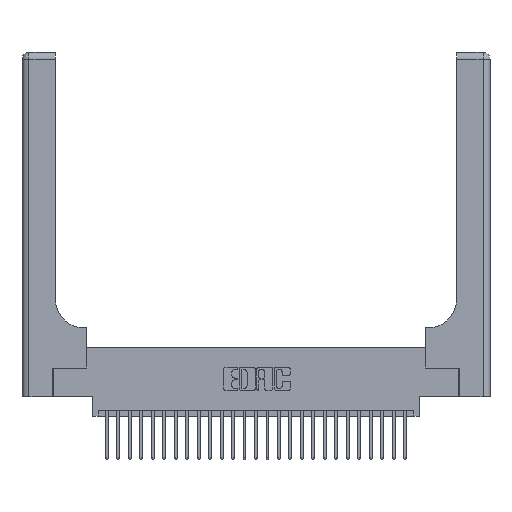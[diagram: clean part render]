
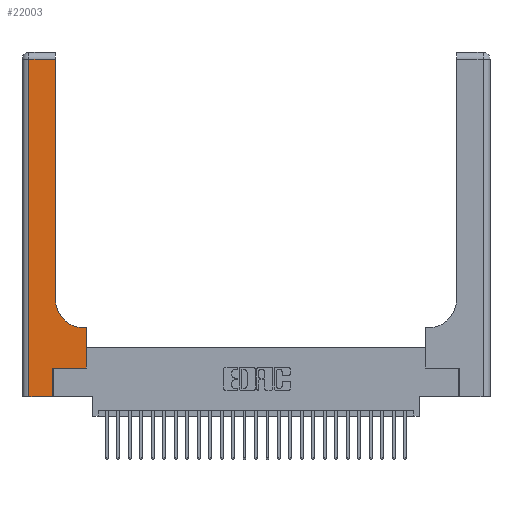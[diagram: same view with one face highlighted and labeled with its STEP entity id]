
A CAD part, top view. The second image highlights one B-rep face of the part: STEP entity #22003.
In plain terms, the highlighted planar face has unit normal (0, 0, 1).
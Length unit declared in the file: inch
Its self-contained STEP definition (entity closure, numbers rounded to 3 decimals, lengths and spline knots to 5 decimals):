
#26 = DIRECTION ( 'NONE',  ( 0., 0., -1. ) ) ;
#573 = CARTESIAN_POINT ( 'NONE',  ( 0.5415, 0.6, 0.37 ) ) ;
#865 = ORIENTED_EDGE ( 'NONE', *, *, #6812, .T. ) ;
#1028 = DIRECTION ( 'NONE',  ( -1., 0., 0. ) ) ;
#1281 = EDGE_CURVE ( 'NONE', #1864, #8788, #22745, .T. ) ;
#1453 = VERTEX_POINT ( 'NONE', #10189 ) ;
#1601 = VECTOR ( 'NONE', #24154, 39.37008 ) ;
#1743 = CARTESIAN_POINT ( 'NONE',  ( 0.2915, 3., 0.37 ) ) ;
#1758 = ORIENTED_EDGE ( 'NONE', *, *, #19657, .T. ) ;
#1864 = VERTEX_POINT ( 'NONE', #3939 ) ;
#1997 = CARTESIAN_POINT ( 'NONE',  ( 0.2915, 2.94, 0.37 ) ) ;
#2528 = LINE ( 'NONE', #7137, #20382 ) ;
#2543 = CARTESIAN_POINT ( 'NONE',  ( 0.269, 0., 0.37 ) ) ;
#3663 = CARTESIAN_POINT ( 'NONE',  ( 0.269, 0., 0.37 ) ) ;
#3703 = CARTESIAN_POINT ( 'NONE',  ( 0.06, 0., 0.37 ) ) ;
#3939 = CARTESIAN_POINT ( 'NONE',  ( 0.5585, 0.6, 0.37 ) ) ;
#4134 = CARTESIAN_POINT ( 'NONE',  ( 0.5415, 0.85, 0.37 ) ) ;
#4213 = EDGE_LOOP ( 'NONE', ( #15264, #865, #1758, #17412, #26661, #13820, #6645, #8659, #6832 ) ) ;
#6259 = CARTESIAN_POINT ( 'NONE',  ( 0.06, 2.94, 0.37 ) ) ;
#6505 = DIRECTION ( 'NONE',  ( -1., 0., 0. ) ) ;
#6563 = VECTOR ( 'NONE', #8230, 39.37008 ) ;
#6645 = ORIENTED_EDGE ( 'NONE', *, *, #28175, .T. ) ;
#6812 = EDGE_CURVE ( 'NONE', #24432, #19133, #2528, .T. ) ;
#6832 = ORIENTED_EDGE ( 'NONE', *, *, #24464, .T. ) ;
#7137 = CARTESIAN_POINT ( 'NONE',  ( 0., 2.94, 0.37 ) ) ;
#7261 = AXIS2_PLACEMENT_3D ( 'NONE', #19276, #26, #6505 ) ;
#7262 = VECTOR ( 'NONE', #17099, 39.37008 ) ;
#7584 = LINE ( 'NONE', #11209, #6563 ) ;
#7883 = DIRECTION ( 'NONE',  ( 0., 1., 0. ) ) ;
#8230 = DIRECTION ( 'NONE',  ( 1., 0., 0. ) ) ;
#8587 = DIRECTION ( 'NONE',  ( 1., 0., 0. ) ) ;
#8659 = ORIENTED_EDGE ( 'NONE', *, *, #1281, .T. ) ;
#8668 = CARTESIAN_POINT ( 'NONE',  ( 0.5585, 0.25, 0.37 ) ) ;
#8682 = CARTESIAN_POINT ( 'NONE',  ( 0., 0., 0.37 ) ) ;
#8788 = VERTEX_POINT ( 'NONE', #573 ) ;
#8790 = EDGE_CURVE ( 'NONE', #1453, #21099, #7584, .T. ) ;
#8958 = LINE ( 'NONE', #16676, #24446 ) ;
#10189 = CARTESIAN_POINT ( 'NONE',  ( 0.269, 0.25, 0.37 ) ) ;
#11209 = CARTESIAN_POINT ( 'NONE',  ( 0.269, 0.25, 0.37 ) ) ;
#12866 = EDGE_CURVE ( 'NONE', #22242, #1453, #25228, .T. ) ;
#13490 = LINE ( 'NONE', #8682, #27992 ) ;
#13820 = ORIENTED_EDGE ( 'NONE', *, *, #8790, .T. ) ;
#14157 = EDGE_CURVE ( 'NONE', #16827, #24432, #25155, .T. ) ;
#14690 = CARTESIAN_POINT ( 'NONE',  ( 0.2915, 0.85, 0.37 ) ) ;
#15157 = DIRECTION ( 'NONE',  ( 1., 0., 0. ) ) ;
#15264 = ORIENTED_EDGE ( 'NONE', *, *, #14157, .T. ) ;
#16146 = CARTESIAN_POINT ( 'NONE',  ( 0.5585, 0.25, 0.37 ) ) ;
#16676 = CARTESIAN_POINT ( 'NONE',  ( 0.06, 3., 0.37 ) ) ;
#16778 = DIRECTION ( 'NONE',  ( 0., -1., 0. ) ) ;
#16827 = VERTEX_POINT ( 'NONE', #14690 ) ;
#16899 = VECTOR ( 'NONE', #1028, 39.37008 ) ;
#17059 = PLANE ( 'NONE',  #7261 ) ;
#17099 = DIRECTION ( 'NONE',  ( 0., 1., 0. ) ) ;
#17341 = DIRECTION ( 'NONE',  ( 0., 0., -1. ) ) ;
#17412 = ORIENTED_EDGE ( 'NONE', *, *, #18472, .T. ) ;
#18472 = EDGE_CURVE ( 'NONE', #27932, #22242, #13490, .T. ) ;
#19133 = VERTEX_POINT ( 'NONE', #6259 ) ;
#19276 = CARTESIAN_POINT ( 'NONE',  ( 0., 3., 0.37 ) ) ;
#19476 = FACE_OUTER_BOUND ( 'NONE', #4213, .T. ) ;
#19657 = EDGE_CURVE ( 'NONE', #19133, #27932, #8958, .T. ) ;
#20382 = VECTOR ( 'NONE', #22488, 39.37008 ) ;
#21099 = VERTEX_POINT ( 'NONE', #16146 ) ;
#22003 = ADVANCED_FACE ( 'NONE', ( #19476 ), #17059, .F. ) ;
#22242 = VERTEX_POINT ( 'NONE', #2543 ) ;
#22488 = DIRECTION ( 'NONE',  ( -1., 0., 0. ) ) ;
#22745 = LINE ( 'NONE', #22947, #16899 ) ;
#22947 = CARTESIAN_POINT ( 'NONE',  ( 0.2915, 0.6, 0.37 ) ) ;
#24154 = DIRECTION ( 'NONE',  ( 0., 1., 0. ) ) ;
#24432 = VERTEX_POINT ( 'NONE', #1997 ) ;
#24446 = VECTOR ( 'NONE', #16778, 39.37008 ) ;
#24464 = EDGE_CURVE ( 'NONE', #8788, #16827, #24901, .T. ) ;
#24901 = CIRCLE ( 'NONE', #27805, 0.25 ) ;
#25155 = LINE ( 'NONE', #1743, #7262 ) ;
#25228 = LINE ( 'NONE', #3663, #26973 ) ;
#26661 = ORIENTED_EDGE ( 'NONE', *, *, #12866, .T. ) ;
#26973 = VECTOR ( 'NONE', #7883, 39.37008 ) ;
#27805 = AXIS2_PLACEMENT_3D ( 'NONE', #4134, #17341, #15157 ) ;
#27932 = VERTEX_POINT ( 'NONE', #3703 ) ;
#27992 = VECTOR ( 'NONE', #8587, 39.37008 ) ;
#28175 = EDGE_CURVE ( 'NONE', #21099, #1864, #28489, .T. ) ;
#28489 = LINE ( 'NONE', #8668, #1601 ) ;
